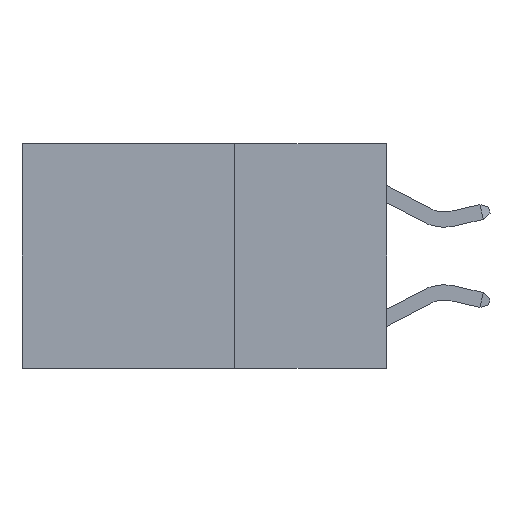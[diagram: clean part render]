
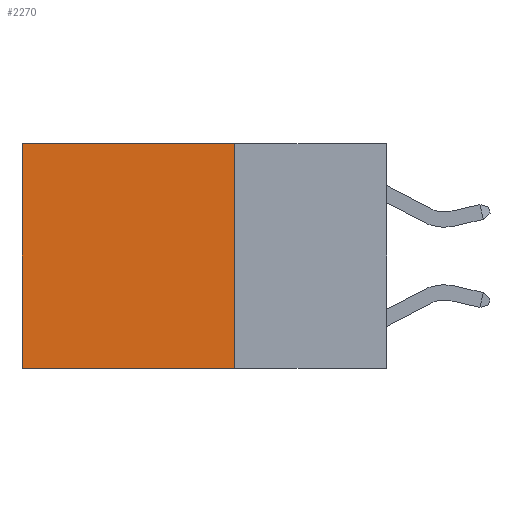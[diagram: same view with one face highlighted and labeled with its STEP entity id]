
A CAD part, left-side view. The second image highlights one B-rep face of the part: STEP entity #2270.
In plain terms, the highlighted planar face has unit normal (-1, 0, 0).
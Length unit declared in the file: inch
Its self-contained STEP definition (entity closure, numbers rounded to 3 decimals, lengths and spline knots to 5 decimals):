
#174 = VECTOR ( 'NONE', #2633, 39.37008 ) ;
#419 = ORIENTED_EDGE ( 'NONE', *, *, #11581, .T. ) ;
#421 = PLANE ( 'NONE',  #9229 ) ;
#673 = VECTOR ( 'NONE', #8970, 39.37008 ) ;
#1013 = EDGE_CURVE ( 'NONE', #5508, #4821, #2682, .T. ) ;
#1066 = ORIENTED_EDGE ( 'NONE', *, *, #1013, .F. ) ;
#1634 = FACE_OUTER_BOUND ( 'NONE', #1755, .T. ) ;
#1755 = EDGE_LOOP ( 'NONE', ( #12213, #9250, #1066, #419 ) ) ;
#2270 = ADVANCED_FACE ( 'NONE', ( #1634 ), #421, .F. ) ;
#2443 = CARTESIAN_POINT ( 'NONE',  ( 0.2625, 0.6, 0. ) ) ;
#2585 = CARTESIAN_POINT ( 'NONE',  ( 0.2625, 0.6, 0. ) ) ;
#2633 = DIRECTION ( 'NONE',  ( 0., 0., -1. ) ) ;
#2682 = LINE ( 'NONE', #8344, #174 ) ;
#4040 = DIRECTION ( 'NONE',  ( 0., 1., 0. ) ) ;
#4189 = LINE ( 'NONE', #2443, #7607 ) ;
#4525 = LINE ( 'NONE', #8931, #673 ) ;
#4821 = VERTEX_POINT ( 'NONE', #6028 ) ;
#5508 = VERTEX_POINT ( 'NONE', #12165 ) ;
#5904 = CARTESIAN_POINT ( 'NONE',  ( 0.2625, 0.25, 0. ) ) ;
#6028 = CARTESIAN_POINT ( 'NONE',  ( 0.2625, 0.25, -0.37 ) ) ;
#6908 = VECTOR ( 'NONE', #4040, 39.37008 ) ;
#7013 = DIRECTION ( 'NONE',  ( 1., 0., 0. ) ) ;
#7607 = VECTOR ( 'NONE', #10175, 39.37008 ) ;
#7959 = VERTEX_POINT ( 'NONE', #9135 ) ;
#8104 = CARTESIAN_POINT ( 'NONE',  ( 0.2625, 0.25, 0. ) ) ;
#8344 = CARTESIAN_POINT ( 'NONE',  ( 0.2625, 0.25, 0. ) ) ;
#8931 = CARTESIAN_POINT ( 'NONE',  ( 0.2625, 0.25, -0.37 ) ) ;
#8970 = DIRECTION ( 'NONE',  ( 0., 1., 0. ) ) ;
#9135 = CARTESIAN_POINT ( 'NONE',  ( 0.2625, 0.6, -0.37 ) ) ;
#9229 = AXIS2_PLACEMENT_3D ( 'NONE', #8104, #7013, #10008 ) ;
#9250 = ORIENTED_EDGE ( 'NONE', *, *, #11734, .F. ) ;
#9462 = VERTEX_POINT ( 'NONE', #2585 ) ;
#10008 = DIRECTION ( 'NONE',  ( 0., 0., -1. ) ) ;
#10059 = EDGE_CURVE ( 'NONE', #9462, #7959, #4189, .T. ) ;
#10175 = DIRECTION ( 'NONE',  ( 0., 0., -1. ) ) ;
#11581 = EDGE_CURVE ( 'NONE', #5508, #9462, #11804, .T. ) ;
#11734 = EDGE_CURVE ( 'NONE', #4821, #7959, #4525, .T. ) ;
#11804 = LINE ( 'NONE', #5904, #6908 ) ;
#12165 = CARTESIAN_POINT ( 'NONE',  ( 0.2625, 0.25, 0. ) ) ;
#12213 = ORIENTED_EDGE ( 'NONE', *, *, #10059, .T. ) ;
